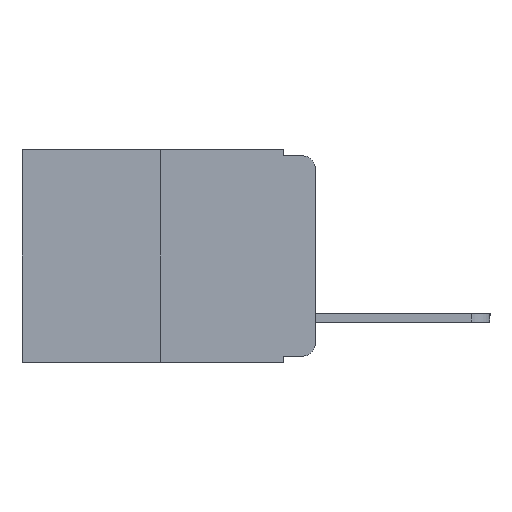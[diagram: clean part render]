
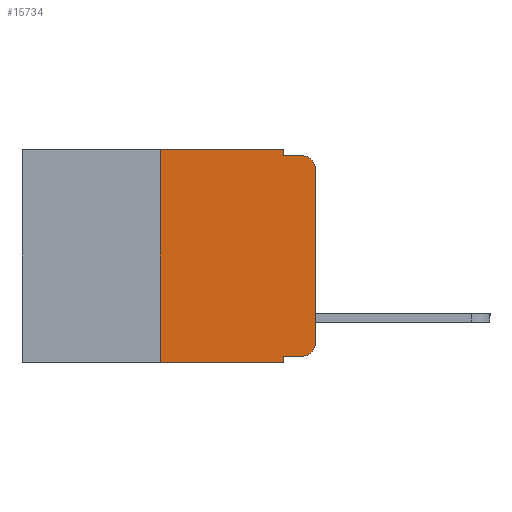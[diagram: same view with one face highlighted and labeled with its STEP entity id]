
A CAD part, left-side view. The second image highlights one B-rep face of the part: STEP entity #15734.
In plain terms, the highlighted planar face has unit normal (-1, 0, 0).
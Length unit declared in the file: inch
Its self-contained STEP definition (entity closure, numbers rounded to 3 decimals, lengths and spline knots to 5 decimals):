
#265 = PLANE ( 'NONE',  #1795 ) ;
#376 = CARTESIAN_POINT ( 'NONE',  ( 0., 0.051, -0.333 ) ) ;
#491 = EDGE_CURVE ( 'NONE', #10084, #11085, #9575, .T. ) ;
#608 = LINE ( 'NONE', #2007, #7009 ) ;
#1083 = CARTESIAN_POINT ( 'NONE',  ( 0., 0., -0.03 ) ) ;
#1341 = EDGE_CURVE ( 'NONE', #14418, #11085, #13697, .T. ) ;
#1542 = DIRECTION ( 'NONE',  ( 1., 0., 0. ) ) ;
#1554 = EDGE_CURVE ( 'NONE', #10097, #2604, #10793, .T. ) ;
#1590 = VECTOR ( 'NONE', #9706, 39.37008 ) ;
#1678 = VECTOR ( 'NONE', #11788, 39.37008 ) ;
#1789 = FACE_OUTER_BOUND ( 'NONE', #2222, .T. ) ;
#1795 = AXIS2_PLACEMENT_3D ( 'NONE', #9086, #1542, #10258 ) ;
#1995 = DIRECTION ( 'NONE',  ( 0., 0., 1. ) ) ;
#2007 = CARTESIAN_POINT ( 'NONE',  ( 0., 0.051, 0. ) ) ;
#2222 = EDGE_LOOP ( 'NONE', ( #2994, #3021, #3094, #3209, #3240, #3302, #3317, #3410, #3428, #3484 ) ) ;
#2479 = VECTOR ( 'NONE', #7589, 39.37008 ) ;
#2604 = VERTEX_POINT ( 'NONE', #8759 ) ;
#2741 = CARTESIAN_POINT ( 'NONE',  ( 0., 0.25, 0. ) ) ;
#2952 = DIRECTION ( 'NONE',  ( 0., 0., 1. ) ) ;
#2994 = ORIENTED_EDGE ( 'NONE', *, *, #3958, .T. ) ;
#3021 = ORIENTED_EDGE ( 'NONE', *, *, #1341, .T. ) ;
#3094 = ORIENTED_EDGE ( 'NONE', *, *, #491, .F. ) ;
#3145 = DIRECTION ( 'NONE',  ( -1., 0., 0. ) ) ;
#3209 = ORIENTED_EDGE ( 'NONE', *, *, #15425, .F. ) ;
#3214 = CARTESIAN_POINT ( 'NONE',  ( 0., 0.02, -0.01 ) ) ;
#3240 = ORIENTED_EDGE ( 'NONE', *, *, #15531, .F. ) ;
#3302 = ORIENTED_EDGE ( 'NONE', *, *, #14673, .F. ) ;
#3317 = ORIENTED_EDGE ( 'NONE', *, *, #1554, .T. ) ;
#3319 = DIRECTION ( 'NONE',  ( 0., 0., -1. ) ) ;
#3410 = ORIENTED_EDGE ( 'NONE', *, *, #13896, .F. ) ;
#3428 = ORIENTED_EDGE ( 'NONE', *, *, #13139, .T. ) ;
#3484 = ORIENTED_EDGE ( 'NONE', *, *, #11570, .T. ) ;
#3565 = CARTESIAN_POINT ( 'NONE',  ( 0., 0.473, -0.343 ) ) ;
#3666 = LINE ( 'NONE', #11496, #6657 ) ;
#3815 = AXIS2_PLACEMENT_3D ( 'NONE', #10502, #3145, #11660 ) ;
#3958 = EDGE_CURVE ( 'NONE', #8300, #14418, #15588, .T. ) ;
#4852 = DIRECTION ( 'NONE',  ( 0., -1., 0. ) ) ;
#4939 = CARTESIAN_POINT ( 'NONE',  ( 0., 0.25, -0.343 ) ) ;
#5262 = CARTESIAN_POINT ( 'NONE',  ( 0., 0.02, -0.333 ) ) ;
#5611 = DIRECTION ( 'NONE',  ( 0., 0., -1. ) ) ;
#5845 = DIRECTION ( 'NONE',  ( -1., 0., 0. ) ) ;
#5858 = CARTESIAN_POINT ( 'NONE',  ( 0., 0.02, -0.03 ) ) ;
#6017 = VERTEX_POINT ( 'NONE', #13405 ) ;
#6150 = VERTEX_POINT ( 'NONE', #2741 ) ;
#6347 = VECTOR ( 'NONE', #13852, 39.37008 ) ;
#6657 = VECTOR ( 'NONE', #2952, 39.37008 ) ;
#7009 = VECTOR ( 'NONE', #3319, 39.37008 ) ;
#7180 = AXIS2_PLACEMENT_3D ( 'NONE', #5858, #5845, #5611 ) ;
#7293 = CARTESIAN_POINT ( 'NONE',  ( 0., 0.473, 0. ) ) ;
#7494 = CIRCLE ( 'NONE', #3815, 0.02 ) ;
#7589 = DIRECTION ( 'NONE',  ( 0., 0., -1. ) ) ;
#7791 = VECTOR ( 'NONE', #4852, 39.37008 ) ;
#8300 = VERTEX_POINT ( 'NONE', #12401 ) ;
#8759 = CARTESIAN_POINT ( 'NONE',  ( 0., 0.051, -0.343 ) ) ;
#8913 = VERTEX_POINT ( 'NONE', #376 ) ;
#9086 = CARTESIAN_POINT ( 'NONE',  ( 0., 0.473, 0. ) ) ;
#9575 = LINE ( 'NONE', #13612, #6347 ) ;
#9706 = DIRECTION ( 'NONE',  ( 0., -1., 0. ) ) ;
#9954 = CARTESIAN_POINT ( 'NONE',  ( 0., 0.051, 0. ) ) ;
#10084 = VERTEX_POINT ( 'NONE', #13247 ) ;
#10097 = VERTEX_POINT ( 'NONE', #4939 ) ;
#10258 = DIRECTION ( 'NONE',  ( 0., 0., -1. ) ) ;
#10502 = CARTESIAN_POINT ( 'NONE',  ( 0., 0.02, -0.313 ) ) ;
#10793 = LINE ( 'NONE', #3565, #1678 ) ;
#10956 = LINE ( 'NONE', #13234, #7791 ) ;
#11085 = VERTEX_POINT ( 'NONE', #3214 ) ;
#11441 = LINE ( 'NONE', #7293, #1590 ) ;
#11496 = CARTESIAN_POINT ( 'NONE',  ( 0., 0.25, 0. ) ) ;
#11570 = EDGE_CURVE ( 'NONE', #14562, #8300, #7494, .T. ) ;
#11660 = DIRECTION ( 'NONE',  ( 0., 0., -1. ) ) ;
#11788 = DIRECTION ( 'NONE',  ( 0., -1., 0. ) ) ;
#12228 = LINE ( 'NONE', #9954, #2479 ) ;
#12401 = CARTESIAN_POINT ( 'NONE',  ( 0., 0., -0.313 ) ) ;
#12562 = VECTOR ( 'NONE', #1995, 39.37008 ) ;
#13139 = EDGE_CURVE ( 'NONE', #8913, #14562, #10956, .T. ) ;
#13234 = CARTESIAN_POINT ( 'NONE',  ( 0., 0.051, -0.333 ) ) ;
#13247 = CARTESIAN_POINT ( 'NONE',  ( 0., 0.051, -0.01 ) ) ;
#13405 = CARTESIAN_POINT ( 'NONE',  ( 0., 0.051, 0. ) ) ;
#13612 = CARTESIAN_POINT ( 'NONE',  ( 0., 0.051, -0.01 ) ) ;
#13697 = CIRCLE ( 'NONE', #7180, 0.02 ) ;
#13852 = DIRECTION ( 'NONE',  ( 0., -1., 0. ) ) ;
#13896 = EDGE_CURVE ( 'NONE', #8913, #2604, #12228, .T. ) ;
#14155 = CARTESIAN_POINT ( 'NONE',  ( 0., 0., 0. ) ) ;
#14418 = VERTEX_POINT ( 'NONE', #1083 ) ;
#14562 = VERTEX_POINT ( 'NONE', #5262 ) ;
#14673 = EDGE_CURVE ( 'NONE', #10097, #6150, #3666, .T. ) ;
#15425 = EDGE_CURVE ( 'NONE', #6017, #10084, #608, .T. ) ;
#15531 = EDGE_CURVE ( 'NONE', #6150, #6017, #11441, .T. ) ;
#15588 = LINE ( 'NONE', #14155, #12562 ) ;
#15734 = ADVANCED_FACE ( 'NONE', ( #1789 ), #265, .F. ) ;
